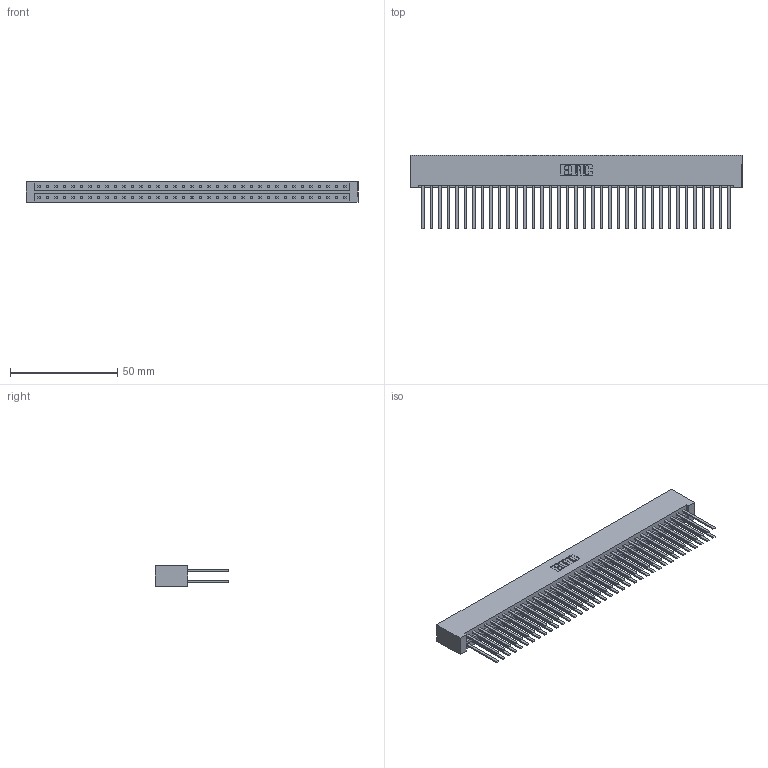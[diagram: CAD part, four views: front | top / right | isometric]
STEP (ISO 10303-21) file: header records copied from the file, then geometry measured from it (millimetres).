
FILE_DESCRIPTION (( 'STEP AP203' ), '1' );
FILE_NAME ('833-074-544-201.STEP', '2020-06-05T16:58:37', ( '' ), ( '' ), 'SwSTEP 2.0', 'SolidWorks 2020', '' );
FILE_SCHEMA (( 'CONFIG_CONTROL_DESIGN' ));
Length unit declared in the file: inch
Products named in the file (3): 833-074-544-201; 345-292-001_345-293-144; 833 Part_Lugless
Assembly tree (75 placements, depth 2):
  833-074-544-201
    833 Part_Lugless
    345-292-001_345-293-144  x74
Bounding box: 154.86 x 34.3 x 9.4 mm (x, y, z)
Volume: 17433.5 mm3; surface area: 23921.4 mm2
Topology: 75 solids, 75 shells, 3510 faces, 10425 edges, 6850 vertices
Faces by surface type: plane 2434, cylinder 1076
Entity records: 23989 total; most frequent: CARTESIAN_POINT 3978, ORIENTED_EDGE 3914, DIRECTION 3397, EDGE_CURVE 1957, LINE 1841, VECTOR 1841, VERTEX_POINT 1302, AXIS2_PLACEMENT_3D 778
